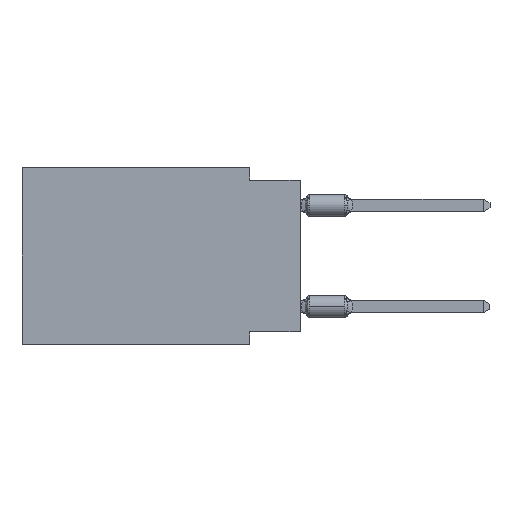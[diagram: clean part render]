
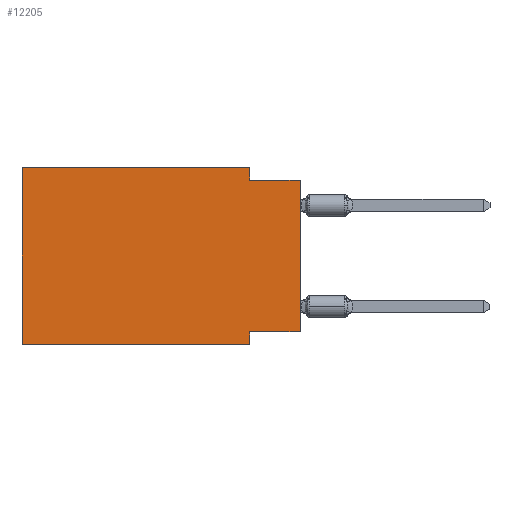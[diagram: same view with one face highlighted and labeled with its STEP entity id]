
A CAD part, left-side view. The second image highlights one B-rep face of the part: STEP entity #12205.
In plain terms, the highlighted planar face has unit normal (-1, 0, 0).
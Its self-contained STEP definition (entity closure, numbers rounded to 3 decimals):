
#762 = ORIENTED_EDGE ( 'NONE', *, *, #9190, .T. ) ;
#993 = VERTEX_POINT ( 'NONE', #18577 ) ;
#1002 = VERTEX_POINT ( 'NONE', #26504 ) ;
#1479 = VERTEX_POINT ( 'NONE', #21452 ) ;
#1583 = EDGE_CURVE ( 'NONE', #993, #6394, #28748, .T. ) ;
#2952 = DIRECTION ( 'NONE',  ( 0., 0., 1. ) ) ;
#2961 = CARTESIAN_POINT ( 'NONE',  ( 0., 2.54, -8.89 ) ) ;
#3217 = VERTEX_POINT ( 'NONE', #17622 ) ;
#3708 = EDGE_CURVE ( 'NONE', #20365, #993, #18442, .T. ) ;
#3821 = LINE ( 'NONE', #26313, #7781 ) ;
#3900 = DIRECTION ( 'NONE',  ( 0., 0., 1. ) ) ;
#4154 = VERTEX_POINT ( 'NONE', #5504 ) ;
#4237 = EDGE_CURVE ( 'NONE', #20365, #3217, #6363, .T. ) ;
#4359 = DIRECTION ( 'NONE',  ( 0., -1., 0. ) ) ;
#4611 = EDGE_LOOP ( 'NONE', ( #762, #19845, #12982, #17724, #5687, #5193, #15118, #28427 ) ) ;
#4991 = VECTOR ( 'NONE', #5159, 1000. ) ;
#5159 = DIRECTION ( 'NONE',  ( 0., 0., -1. ) ) ;
#5193 = ORIENTED_EDGE ( 'NONE', *, *, #4237, .T. ) ;
#5504 = CARTESIAN_POINT ( 'NONE',  ( 0., 0., -0.635 ) ) ;
#5687 = ORIENTED_EDGE ( 'NONE', *, *, #3708, .F. ) ;
#6363 = LINE ( 'NONE', #17343, #15301 ) ;
#6394 = VERTEX_POINT ( 'NONE', #17559 ) ;
#7671 = VECTOR ( 'NONE', #4359, 1000. ) ;
#7781 = VECTOR ( 'NONE', #21943, 1000. ) ;
#9190 = EDGE_CURVE ( 'NONE', #1002, #4154, #24357, .T. ) ;
#10448 = CARTESIAN_POINT ( 'NONE',  ( 0., 13.97, 0. ) ) ;
#10830 = CARTESIAN_POINT ( 'NONE',  ( 0., 0., -8.255 ) ) ;
#11062 = CARTESIAN_POINT ( 'NONE',  ( 0., 0., 0. ) ) ;
#12168 = VECTOR ( 'NONE', #3900, 1000. ) ;
#12205 = ADVANCED_FACE ( 'NONE', ( #14568 ), #18962, .F. ) ;
#12934 = VECTOR ( 'NONE', #2952, 1000. ) ;
#12982 = ORIENTED_EDGE ( 'NONE', *, *, #19711, .F. ) ;
#13008 = LINE ( 'NONE', #10830, #16518 ) ;
#13081 = DIRECTION ( 'NONE',  ( 0., -1., 0. ) ) ;
#13700 = EDGE_CURVE ( 'NONE', #1479, #4154, #19858, .T. ) ;
#14568 = FACE_OUTER_BOUND ( 'NONE', #4611, .T. ) ;
#14662 = VECTOR ( 'NONE', #14871, 1000. ) ;
#14871 = DIRECTION ( 'NONE',  ( 0., -1., 0. ) ) ;
#15118 = ORIENTED_EDGE ( 'NONE', *, *, #19634, .F. ) ;
#15301 = VECTOR ( 'NONE', #13081, 1000. ) ;
#16518 = VECTOR ( 'NONE', #21638, 1000. ) ;
#17044 = DIRECTION ( 'NONE',  ( 1., 0., 0. ) ) ;
#17343 = CARTESIAN_POINT ( 'NONE',  ( 0., 13.97, -8.89 ) ) ;
#17559 = CARTESIAN_POINT ( 'NONE',  ( 0., 2.54, 0. ) ) ;
#17622 = CARTESIAN_POINT ( 'NONE',  ( 0., 2.54, -8.89 ) ) ;
#17724 = ORIENTED_EDGE ( 'NONE', *, *, #1583, .F. ) ;
#18442 = LINE ( 'NONE', #27923, #12934 ) ;
#18577 = CARTESIAN_POINT ( 'NONE',  ( 0., 13.97, 0. ) ) ;
#18938 = CARTESIAN_POINT ( 'NONE',  ( 0., 2.54, -8.255 ) ) ;
#18962 = PLANE ( 'NONE',  #28803 ) ;
#19634 = EDGE_CURVE ( 'NONE', #22417, #3217, #27652, .T. ) ;
#19711 = EDGE_CURVE ( 'NONE', #6394, #1479, #3821, .T. ) ;
#19842 = CARTESIAN_POINT ( 'NONE',  ( 0., 13.97, 0. ) ) ;
#19845 = ORIENTED_EDGE ( 'NONE', *, *, #13700, .F. ) ;
#19858 = LINE ( 'NONE', #24374, #7671 ) ;
#20365 = VERTEX_POINT ( 'NONE', #23794 ) ;
#21219 = EDGE_CURVE ( 'NONE', #1002, #22417, #13008, .T. ) ;
#21452 = CARTESIAN_POINT ( 'NONE',  ( 0., 2.54, -0.635 ) ) ;
#21638 = DIRECTION ( 'NONE',  ( 0., 1., 0. ) ) ;
#21943 = DIRECTION ( 'NONE',  ( 0., 0., -1. ) ) ;
#22417 = VERTEX_POINT ( 'NONE', #18938 ) ;
#23794 = CARTESIAN_POINT ( 'NONE',  ( 0., 13.97, -8.89 ) ) ;
#24357 = LINE ( 'NONE', #11062, #12168 ) ;
#24374 = CARTESIAN_POINT ( 'NONE',  ( 0., 0., -0.635 ) ) ;
#25947 = DIRECTION ( 'NONE',  ( 0., 0., -1. ) ) ;
#26313 = CARTESIAN_POINT ( 'NONE',  ( 0., 2.54, 0. ) ) ;
#26504 = CARTESIAN_POINT ( 'NONE',  ( 0., 0., -8.255 ) ) ;
#27652 = LINE ( 'NONE', #2961, #4991 ) ;
#27923 = CARTESIAN_POINT ( 'NONE',  ( 0., 13.97, 0. ) ) ;
#28427 = ORIENTED_EDGE ( 'NONE', *, *, #21219, .F. ) ;
#28748 = LINE ( 'NONE', #19842, #14662 ) ;
#28803 = AXIS2_PLACEMENT_3D ( 'NONE', #10448, #17044, #25947 ) ;
